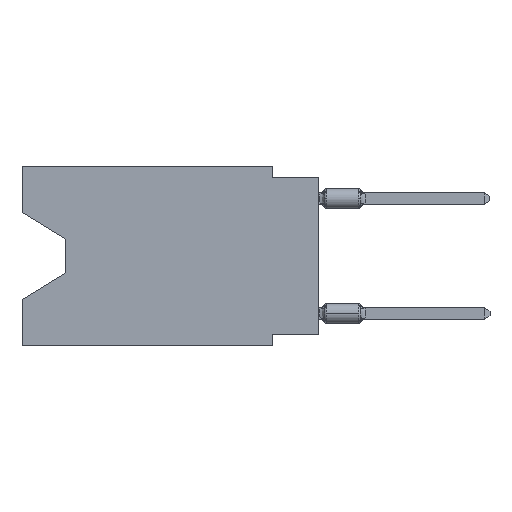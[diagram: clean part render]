
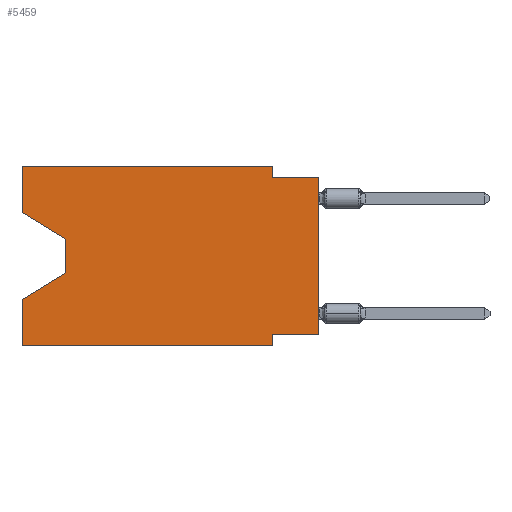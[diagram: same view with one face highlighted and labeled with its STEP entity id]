
A CAD part, left-side view. The second image highlights one B-rep face of the part: STEP entity #5459.
In plain terms, the highlighted planar face has unit normal (-1, 0, 0).
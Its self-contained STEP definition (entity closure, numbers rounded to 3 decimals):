
#26 = VECTOR ( 'NONE', #16864, 1000. ) ;
#65 = CARTESIAN_POINT ( 'NONE',  ( 0., 16.383, 0. ) ) ;
#193 = EDGE_CURVE ( 'NONE', #2659, #644, #11082, .T. ) ;
#234 = DIRECTION ( 'NONE',  ( 0., 0.855, -0.519 ) ) ;
#334 = AXIS2_PLACEMENT_3D ( 'NONE', #4169, #9017, #14777 ) ;
#644 = VERTEX_POINT ( 'NONE', #12596 ) ;
#894 = EDGE_CURVE ( 'NONE', #17967, #12092, #12011, .T. ) ;
#1294 = CARTESIAN_POINT ( 'NONE',  ( 0., 0., -9.271 ) ) ;
#1376 = CARTESIAN_POINT ( 'NONE',  ( 0., 16.383, -9.906 ) ) ;
#1557 = CARTESIAN_POINT ( 'NONE',  ( 0., 13.97, -5.893 ) ) ;
#1779 = EDGE_CURVE ( 'NONE', #2449, #16385, #9695, .T. ) ;
#1840 = CARTESIAN_POINT ( 'NONE',  ( 0., 2.54, -9.271 ) ) ;
#1854 = VECTOR ( 'NONE', #12204, 1000. ) ;
#1876 = PLANE ( 'NONE',  #334 ) ;
#2022 = EDGE_CURVE ( 'NONE', #7484, #8648, #9978, .T. ) ;
#2336 = ORIENTED_EDGE ( 'NONE', *, *, #1779, .F. ) ;
#2342 = VECTOR ( 'NONE', #4186, 1000. ) ;
#2434 = EDGE_CURVE ( 'NONE', #7909, #16176, #13043, .T. ) ;
#2443 = VECTOR ( 'NONE', #17063, 1000. ) ;
#2449 = VERTEX_POINT ( 'NONE', #1840 ) ;
#2659 = VERTEX_POINT ( 'NONE', #6923 ) ;
#3194 = LINE ( 'NONE', #13257, #2443 ) ;
#3223 = ORIENTED_EDGE ( 'NONE', *, *, #193, .F. ) ;
#3262 = ORIENTED_EDGE ( 'NONE', *, *, #5499, .F. ) ;
#3821 = CARTESIAN_POINT ( 'NONE',  ( 0., 16.383, -7.36 ) ) ;
#4169 = CARTESIAN_POINT ( 'NONE',  ( 0., 16.383, 0. ) ) ;
#4186 = DIRECTION ( 'NONE',  ( 0., -0.855, -0.519 ) ) ;
#4373 = LINE ( 'NONE', #1294, #12222 ) ;
#4383 = CARTESIAN_POINT ( 'NONE',  ( 0., 2.54, -0.635 ) ) ;
#4599 = FACE_OUTER_BOUND ( 'NONE', #7159, .T. ) ;
#4615 = VECTOR ( 'NONE', #234, 1000. ) ;
#5299 = CARTESIAN_POINT ( 'NONE',  ( 0., 16.383, 0. ) ) ;
#5392 = CARTESIAN_POINT ( 'NONE',  ( 0., 0., 0. ) ) ;
#5455 = EDGE_CURVE ( 'NONE', #644, #12825, #12448, .T. ) ;
#5459 = ADVANCED_FACE ( 'NONE', ( #4599 ), #1876, .F. ) ;
#5499 = EDGE_CURVE ( 'NONE', #12825, #7484, #3194, .T. ) ;
#5532 = CARTESIAN_POINT ( 'NONE',  ( 0., 16.383, 0. ) ) ;
#5779 = CARTESIAN_POINT ( 'NONE',  ( 0., 16.383, -2.546 ) ) ;
#6690 = CARTESIAN_POINT ( 'NONE',  ( 0., 2.54, 0. ) ) ;
#6729 = CARTESIAN_POINT ( 'NONE',  ( 0., 16.383, -9.906 ) ) ;
#6923 = CARTESIAN_POINT ( 'NONE',  ( 0., 16.383, -2.546 ) ) ;
#7159 = EDGE_LOOP ( 'NONE', ( #8776, #16982, #15363, #15772, #11715, #2336, #16845, #14998, #18105, #3262, #8940, #3223 ) ) ;
#7304 = LINE ( 'NONE', #5779, #2342 ) ;
#7484 = VERTEX_POINT ( 'NONE', #4383 ) ;
#7744 = CARTESIAN_POINT ( 'NONE',  ( 0., 0., -9.271 ) ) ;
#7792 = DIRECTION ( 'NONE',  ( 0., 0., -1. ) ) ;
#7909 = VERTEX_POINT ( 'NONE', #6729 ) ;
#8151 = VECTOR ( 'NONE', #15652, 1000. ) ;
#8511 = VECTOR ( 'NONE', #7792, 1000. ) ;
#8584 = LINE ( 'NONE', #5392, #16704 ) ;
#8609 = LINE ( 'NONE', #1557, #4615 ) ;
#8648 = VERTEX_POINT ( 'NONE', #12375 ) ;
#8776 = ORIENTED_EDGE ( 'NONE', *, *, #13830, .T. ) ;
#8940 = ORIENTED_EDGE ( 'NONE', *, *, #5455, .F. ) ;
#9017 = DIRECTION ( 'NONE',  ( 1., 0., 0. ) ) ;
#9379 = VECTOR ( 'NONE', #17015, 1000. ) ;
#9695 = LINE ( 'NONE', #16681, #26 ) ;
#9978 = LINE ( 'NONE', #10600, #1854 ) ;
#10038 = EDGE_CURVE ( 'NONE', #18172, #2449, #4373, .T. ) ;
#10159 = CARTESIAN_POINT ( 'NONE',  ( 0., 13.97, -5.893 ) ) ;
#10400 = EDGE_CURVE ( 'NONE', #18172, #8648, #8584, .T. ) ;
#10600 = CARTESIAN_POINT ( 'NONE',  ( 0., 0., -0.635 ) ) ;
#11082 = LINE ( 'NONE', #5532, #9379 ) ;
#11715 = ORIENTED_EDGE ( 'NONE', *, *, #13820, .T. ) ;
#12011 = LINE ( 'NONE', #16353, #8511 ) ;
#12092 = VERTEX_POINT ( 'NONE', #10159 ) ;
#12204 = DIRECTION ( 'NONE',  ( 0., -1., 0. ) ) ;
#12222 = VECTOR ( 'NONE', #18489, 1000. ) ;
#12375 = CARTESIAN_POINT ( 'NONE',  ( 0., 0., -0.635 ) ) ;
#12448 = LINE ( 'NONE', #5299, #8151 ) ;
#12596 = CARTESIAN_POINT ( 'NONE',  ( 0., 16.383, 0. ) ) ;
#12825 = VERTEX_POINT ( 'NONE', #6690 ) ;
#13025 = DIRECTION ( 'NONE',  ( 0., -1., 0. ) ) ;
#13043 = LINE ( 'NONE', #65, #17197 ) ;
#13257 = CARTESIAN_POINT ( 'NONE',  ( 0., 2.54, 0. ) ) ;
#13282 = CARTESIAN_POINT ( 'NONE',  ( 0., 13.97, -4.013 ) ) ;
#13820 = EDGE_CURVE ( 'NONE', #7909, #16385, #14271, .T. ) ;
#13830 = EDGE_CURVE ( 'NONE', #2659, #17967, #7304, .T. ) ;
#14271 = LINE ( 'NONE', #1376, #18552 ) ;
#14353 = DIRECTION ( 'NONE',  ( 0., 0., 1. ) ) ;
#14642 = CARTESIAN_POINT ( 'NONE',  ( 0., 2.54, -9.906 ) ) ;
#14777 = DIRECTION ( 'NONE',  ( 0., 0., -1. ) ) ;
#14998 = ORIENTED_EDGE ( 'NONE', *, *, #10400, .T. ) ;
#15363 = ORIENTED_EDGE ( 'NONE', *, *, #16476, .T. ) ;
#15652 = DIRECTION ( 'NONE',  ( 0., -1., 0. ) ) ;
#15772 = ORIENTED_EDGE ( 'NONE', *, *, #2434, .F. ) ;
#15782 = DIRECTION ( 'NONE',  ( 0., 0., 1. ) ) ;
#16176 = VERTEX_POINT ( 'NONE', #3821 ) ;
#16353 = CARTESIAN_POINT ( 'NONE',  ( 0., 13.97, -4.013 ) ) ;
#16385 = VERTEX_POINT ( 'NONE', #14642 ) ;
#16476 = EDGE_CURVE ( 'NONE', #12092, #16176, #8609, .T. ) ;
#16681 = CARTESIAN_POINT ( 'NONE',  ( 0., 2.54, -9.906 ) ) ;
#16704 = VECTOR ( 'NONE', #14353, 1000. ) ;
#16845 = ORIENTED_EDGE ( 'NONE', *, *, #10038, .F. ) ;
#16864 = DIRECTION ( 'NONE',  ( 0., 0., -1. ) ) ;
#16982 = ORIENTED_EDGE ( 'NONE', *, *, #894, .T. ) ;
#17015 = DIRECTION ( 'NONE',  ( 0., 0., 1. ) ) ;
#17063 = DIRECTION ( 'NONE',  ( 0., 0., -1. ) ) ;
#17197 = VECTOR ( 'NONE', #15782, 1000. ) ;
#17967 = VERTEX_POINT ( 'NONE', #13282 ) ;
#18105 = ORIENTED_EDGE ( 'NONE', *, *, #2022, .F. ) ;
#18172 = VERTEX_POINT ( 'NONE', #7744 ) ;
#18489 = DIRECTION ( 'NONE',  ( 0., 1., 0. ) ) ;
#18552 = VECTOR ( 'NONE', #13025, 1000. ) ;
